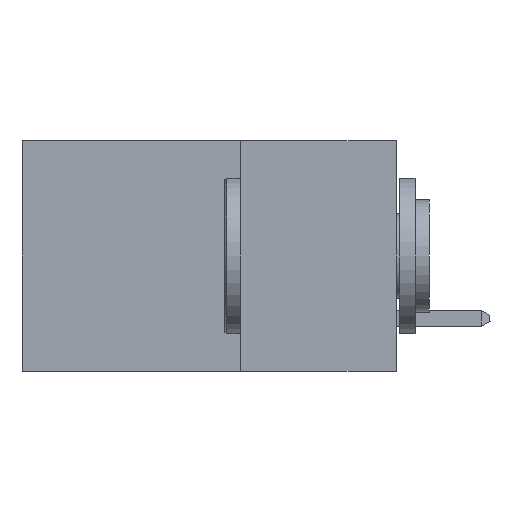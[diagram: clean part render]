
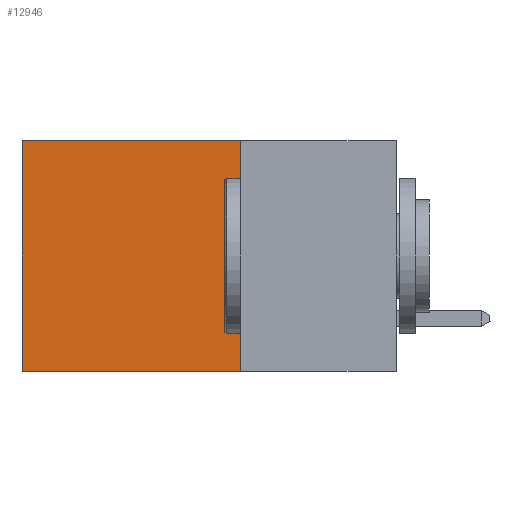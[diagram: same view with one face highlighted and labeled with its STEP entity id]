
A CAD part, left-side view. The second image highlights one B-rep face of the part: STEP entity #12946.
In plain terms, the highlighted planar face has unit normal (-1, 0, 0).
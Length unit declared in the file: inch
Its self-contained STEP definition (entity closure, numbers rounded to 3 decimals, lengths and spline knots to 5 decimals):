
#188 = LINE ( 'NONE', #20047, #11924 ) ;
#377 = CARTESIAN_POINT ( 'NONE',  ( 0.298, 0.25, 0. ) ) ;
#1695 = VECTOR ( 'NONE', #24028, 39.37008 ) ;
#2213 = CARTESIAN_POINT ( 'NONE',  ( 0.298, 0.25, 0. ) ) ;
#4610 = EDGE_CURVE ( 'NONE', #9005, #11336, #13118, .T. ) ;
#5663 = CARTESIAN_POINT ( 'NONE',  ( 0.298, 0.25, -0.37 ) ) ;
#7472 = EDGE_CURVE ( 'NONE', #24134, #11336, #188, .T. ) ;
#7616 = LINE ( 'NONE', #2213, #1695 ) ;
#8251 = CARTESIAN_POINT ( 'NONE',  ( 0.298, 0.25, -0.37 ) ) ;
#9005 = VERTEX_POINT ( 'NONE', #8251 ) ;
#9295 = VERTEX_POINT ( 'NONE', #377 ) ;
#9641 = LINE ( 'NONE', #21382, #21146 ) ;
#10282 = AXIS2_PLACEMENT_3D ( 'NONE', #25674, #27853, #14913 ) ;
#11336 = VERTEX_POINT ( 'NONE', #20365 ) ;
#11924 = VECTOR ( 'NONE', #22226, 39.37008 ) ;
#12946 = ADVANCED_FACE ( 'NONE', ( #26478 ), #23504, .F. ) ;
#13118 = LINE ( 'NONE', #5663, #18838 ) ;
#14041 = ORIENTED_EDGE ( 'NONE', *, *, #16401, .T. ) ;
#14603 = ORIENTED_EDGE ( 'NONE', *, *, #28206, .F. ) ;
#14869 = DIRECTION ( 'NONE',  ( 0., 1., 0. ) ) ;
#14913 = DIRECTION ( 'NONE',  ( 0., 0., -1. ) ) ;
#16401 = EDGE_CURVE ( 'NONE', #9295, #24134, #9641, .T. ) ;
#18838 = VECTOR ( 'NONE', #20873, 39.37008 ) ;
#20047 = CARTESIAN_POINT ( 'NONE',  ( 0.298, 0.6, 0. ) ) ;
#20365 = CARTESIAN_POINT ( 'NONE',  ( 0.298, 0.6, -0.37 ) ) ;
#20873 = DIRECTION ( 'NONE',  ( 0., 1., 0. ) ) ;
#21146 = VECTOR ( 'NONE', #14869, 39.37008 ) ;
#21382 = CARTESIAN_POINT ( 'NONE',  ( 0.298, 0.25, 0. ) ) ;
#22226 = DIRECTION ( 'NONE',  ( 0., 0., -1. ) ) ;
#22927 = ORIENTED_EDGE ( 'NONE', *, *, #4610, .F. ) ;
#23504 = PLANE ( 'NONE',  #10282 ) ;
#24028 = DIRECTION ( 'NONE',  ( 0., 0., -1. ) ) ;
#24134 = VERTEX_POINT ( 'NONE', #24561 ) ;
#24561 = CARTESIAN_POINT ( 'NONE',  ( 0.298, 0.6, 0. ) ) ;
#25674 = CARTESIAN_POINT ( 'NONE',  ( 0.298, 0.25, 0. ) ) ;
#26052 = ORIENTED_EDGE ( 'NONE', *, *, #7472, .T. ) ;
#26478 = FACE_OUTER_BOUND ( 'NONE', #27475, .T. ) ;
#27475 = EDGE_LOOP ( 'NONE', ( #26052, #22927, #14603, #14041 ) ) ;
#27853 = DIRECTION ( 'NONE',  ( 1., 0., 0. ) ) ;
#28206 = EDGE_CURVE ( 'NONE', #9295, #9005, #7616, .T. ) ;
